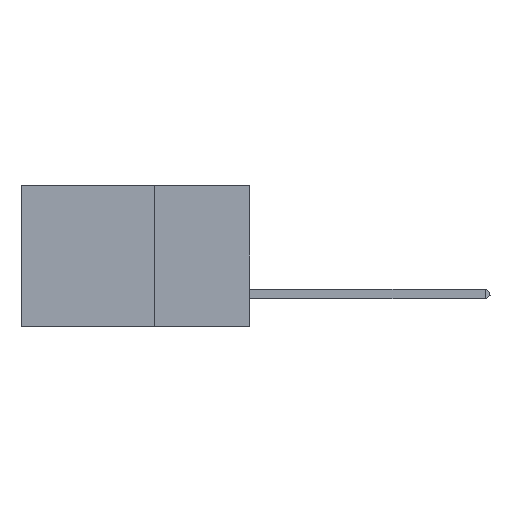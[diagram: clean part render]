
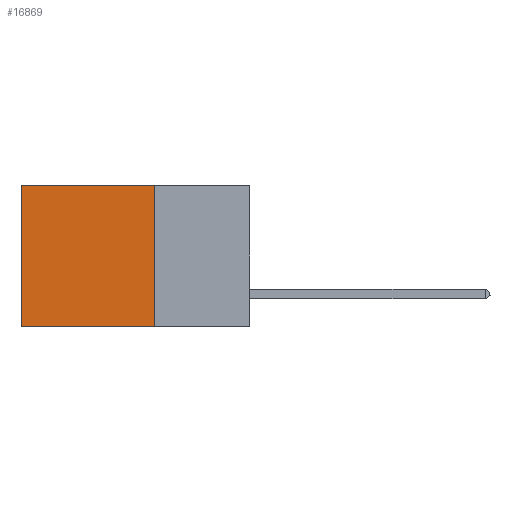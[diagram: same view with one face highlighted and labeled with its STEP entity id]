
A CAD part, left-side view. The second image highlights one B-rep face of the part: STEP entity #16869.
In plain terms, the highlighted planar face has unit normal (-1, 0, 0).
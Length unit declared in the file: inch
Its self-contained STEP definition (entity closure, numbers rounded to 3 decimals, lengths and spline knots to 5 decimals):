
#845 = CARTESIAN_POINT ( 'NONE',  ( 0.2875, 0.25, 0. ) ) ;
#1203 = LINE ( 'NONE', #845, #25250 ) ;
#1582 = DIRECTION ( 'NONE',  ( 0., 0., -1. ) ) ;
#2931 = VERTEX_POINT ( 'NONE', #34242 ) ;
#4074 = DIRECTION ( 'NONE',  ( 1., 0., 0. ) ) ;
#4246 = CARTESIAN_POINT ( 'NONE',  ( 0.2875, 0.25, 0. ) ) ;
#4789 = EDGE_CURVE ( 'NONE', #2931, #27083, #33393, .T. ) ;
#5671 = VERTEX_POINT ( 'NONE', #12449 ) ;
#6378 = DIRECTION ( 'NONE',  ( 0., 1., 0. ) ) ;
#7779 = CARTESIAN_POINT ( 'NONE',  ( 0.2875, 0.6, 0. ) ) ;
#8122 = LINE ( 'NONE', #7779, #28787 ) ;
#9034 = CARTESIAN_POINT ( 'NONE',  ( 0.2875, 0.25, -0.37 ) ) ;
#9073 = EDGE_CURVE ( 'NONE', #5671, #18306, #32538, .T. ) ;
#11025 = EDGE_CURVE ( 'NONE', #5671, #2931, #1203, .T. ) ;
#12449 = CARTESIAN_POINT ( 'NONE',  ( 0.2875, 0.25, 0. ) ) ;
#12474 = AXIS2_PLACEMENT_3D ( 'NONE', #4246, #4074, #1582 ) ;
#15492 = EDGE_LOOP ( 'NONE', ( #20811, #30288, #27876, #31640 ) ) ;
#16869 = ADVANCED_FACE ( 'NONE', ( #30903 ), #28582, .F. ) ;
#18306 = VERTEX_POINT ( 'NONE', #24565 ) ;
#19110 = DIRECTION ( 'NONE',  ( 0., 0., -1. ) ) ;
#20811 = ORIENTED_EDGE ( 'NONE', *, *, #34077, .T. ) ;
#22038 = CARTESIAN_POINT ( 'NONE',  ( 0.2875, 0.25, 0. ) ) ;
#22309 = VECTOR ( 'NONE', #30582, 39.37008 ) ;
#22860 = DIRECTION ( 'NONE',  ( 0., 0., -1. ) ) ;
#24146 = CARTESIAN_POINT ( 'NONE',  ( 0.2875, 0.6, -0.37 ) ) ;
#24565 = CARTESIAN_POINT ( 'NONE',  ( 0.2875, 0.6, 0. ) ) ;
#25250 = VECTOR ( 'NONE', #22860, 39.37008 ) ;
#27083 = VERTEX_POINT ( 'NONE', #24146 ) ;
#27876 = ORIENTED_EDGE ( 'NONE', *, *, #11025, .F. ) ;
#28582 = PLANE ( 'NONE',  #12474 ) ;
#28787 = VECTOR ( 'NONE', #19110, 39.37008 ) ;
#28995 = VECTOR ( 'NONE', #6378, 39.37008 ) ;
#30288 = ORIENTED_EDGE ( 'NONE', *, *, #4789, .F. ) ;
#30582 = DIRECTION ( 'NONE',  ( 0., 1., 0. ) ) ;
#30903 = FACE_OUTER_BOUND ( 'NONE', #15492, .T. ) ;
#31640 = ORIENTED_EDGE ( 'NONE', *, *, #9073, .T. ) ;
#32538 = LINE ( 'NONE', #22038, #22309 ) ;
#33393 = LINE ( 'NONE', #9034, #28995 ) ;
#34077 = EDGE_CURVE ( 'NONE', #18306, #27083, #8122, .T. ) ;
#34242 = CARTESIAN_POINT ( 'NONE',  ( 0.2875, 0.25, -0.37 ) ) ;
